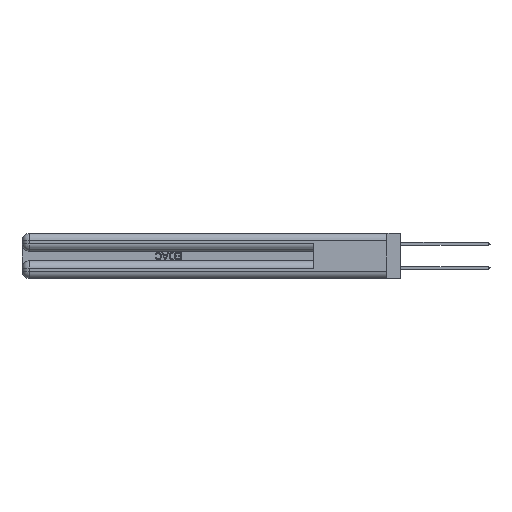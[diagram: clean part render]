
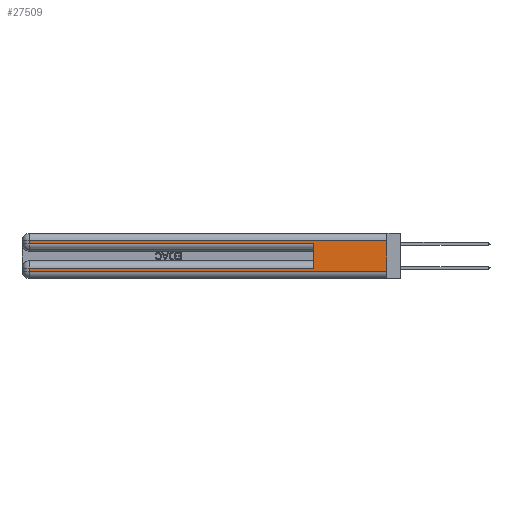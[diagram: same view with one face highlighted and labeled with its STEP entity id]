
A CAD part, left-side view. The second image highlights one B-rep face of the part: STEP entity #27509.
In plain terms, the highlighted planar face has unit normal (-1, 0, 0).
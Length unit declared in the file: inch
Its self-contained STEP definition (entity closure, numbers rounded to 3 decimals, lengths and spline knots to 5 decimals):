
#192 = VERTEX_POINT ( 'NONE', #6987 ) ;
#917 = ORIENTED_EDGE ( 'NONE', *, *, #10895, .T. ) ;
#2391 = CARTESIAN_POINT ( 'NONE',  ( 0., 0., 0.37 ) ) ;
#2930 = VERTEX_POINT ( 'NONE', #15470 ) ;
#3002 = CARTESIAN_POINT ( 'NONE',  ( 0., 0., 0.06 ) ) ;
#3645 = CARTESIAN_POINT ( 'NONE',  ( 0., 0., 0.31 ) ) ;
#3798 = ORIENTED_EDGE ( 'NONE', *, *, #39941, .F. ) ;
#5053 = VECTOR ( 'NONE', #23461, 39.37008 ) ;
#6502 = EDGE_CURVE ( 'NONE', #22265, #192, #21570, .T. ) ;
#6736 = VECTOR ( 'NONE', #7463, 39.37008 ) ;
#6833 = CARTESIAN_POINT ( 'NONE',  ( 0., 2.94, 0.37 ) ) ;
#6987 = CARTESIAN_POINT ( 'NONE',  ( 0., 2.94, 0.285 ) ) ;
#7341 = VERTEX_POINT ( 'NONE', #17289 ) ;
#7463 = DIRECTION ( 'NONE',  ( 0., 1., 0. ) ) ;
#7675 = CARTESIAN_POINT ( 'NONE',  ( 0., 2.94, 0.37 ) ) ;
#8107 = PLANE ( 'NONE',  #39879 ) ;
#8289 = EDGE_CURVE ( 'NONE', #192, #41478, #34525, .T. ) ;
#10895 = EDGE_CURVE ( 'NONE', #2930, #25895, #14862, .T. ) ;
#11434 = DIRECTION ( 'NONE',  ( 0., 0., -1. ) ) ;
#11670 = VECTOR ( 'NONE', #47206, 39.37008 ) ;
#13680 = VECTOR ( 'NONE', #32688, 39.37008 ) ;
#13960 = VERTEX_POINT ( 'NONE', #19303 ) ;
#14805 = ORIENTED_EDGE ( 'NONE', *, *, #6502, .T. ) ;
#14862 = LINE ( 'NONE', #3002, #13680 ) ;
#15470 = CARTESIAN_POINT ( 'NONE',  ( 0., 2.94, 0.06 ) ) ;
#15638 = CARTESIAN_POINT ( 'NONE',  ( 0., 0., 0.37 ) ) ;
#15807 = VECTOR ( 'NONE', #43833, 39.37008 ) ;
#17210 = EDGE_CURVE ( 'NONE', #13960, #41478, #32403, .T. ) ;
#17289 = CARTESIAN_POINT ( 'NONE',  ( 0., 0., 0.31 ) ) ;
#17436 = DIRECTION ( 'NONE',  ( 0., 0., 1. ) ) ;
#19303 = CARTESIAN_POINT ( 'NONE',  ( 0., 0.6, 0.085 ) ) ;
#19344 = DIRECTION ( 'NONE',  ( 1., 0., 0. ) ) ;
#19757 = CARTESIAN_POINT ( 'NONE',  ( 0., 0., 0.285 ) ) ;
#21570 = LINE ( 'NONE', #6833, #11670 ) ;
#22265 = VERTEX_POINT ( 'NONE', #40867 ) ;
#22826 = EDGE_CURVE ( 'NONE', #13960, #40471, #25610, .T. ) ;
#23461 = DIRECTION ( 'NONE',  ( 0., -1., 0. ) ) ;
#24745 = DIRECTION ( 'NONE',  ( 0., 0., -1. ) ) ;
#24899 = ORIENTED_EDGE ( 'NONE', *, *, #30903, .T. ) ;
#24969 = CARTESIAN_POINT ( 'NONE',  ( 0., 0.6, 0.145 ) ) ;
#25610 = LINE ( 'NONE', #32856, #15807 ) ;
#25895 = VERTEX_POINT ( 'NONE', #39810 ) ;
#27509 = ADVANCED_FACE ( 'NONE', ( #47168 ), #8107, .F. ) ;
#28100 = VECTOR ( 'NONE', #24745, 39.37008 ) ;
#29808 = LINE ( 'NONE', #7675, #38330 ) ;
#30903 = EDGE_CURVE ( 'NONE', #40471, #2930, #29808, .T. ) ;
#31263 = VECTOR ( 'NONE', #17436, 39.37008 ) ;
#32403 = LINE ( 'NONE', #24969, #31263 ) ;
#32688 = DIRECTION ( 'NONE',  ( 0., -1., 0. ) ) ;
#32705 = EDGE_LOOP ( 'NONE', ( #3798, #37897, #14805, #44655, #41698, #47774, #24899, #917 ) ) ;
#32856 = CARTESIAN_POINT ( 'NONE',  ( 0., 0., 0.085 ) ) ;
#34525 = LINE ( 'NONE', #19757, #5053 ) ;
#36173 = LINE ( 'NONE', #3645, #6736 ) ;
#36629 = LINE ( 'NONE', #2391, #28100 ) ;
#37897 = ORIENTED_EDGE ( 'NONE', *, *, #38825, .T. ) ;
#38330 = VECTOR ( 'NONE', #11434, 39.37008 ) ;
#38825 = EDGE_CURVE ( 'NONE', #7341, #22265, #36173, .T. ) ;
#39810 = CARTESIAN_POINT ( 'NONE',  ( 0., 0., 0.06 ) ) ;
#39879 = AXIS2_PLACEMENT_3D ( 'NONE', #15638, #19344, #44909 ) ;
#39941 = EDGE_CURVE ( 'NONE', #7341, #25895, #36629, .T. ) ;
#40471 = VERTEX_POINT ( 'NONE', #45754 ) ;
#40763 = CARTESIAN_POINT ( 'NONE',  ( 0., 0.6, 0.285 ) ) ;
#40867 = CARTESIAN_POINT ( 'NONE',  ( 0., 2.94, 0.31 ) ) ;
#41478 = VERTEX_POINT ( 'NONE', #40763 ) ;
#41698 = ORIENTED_EDGE ( 'NONE', *, *, #17210, .F. ) ;
#43833 = DIRECTION ( 'NONE',  ( 0., 1., 0. ) ) ;
#44655 = ORIENTED_EDGE ( 'NONE', *, *, #8289, .T. ) ;
#44909 = DIRECTION ( 'NONE',  ( 0., 0., -1. ) ) ;
#45754 = CARTESIAN_POINT ( 'NONE',  ( 0., 2.94, 0.085 ) ) ;
#47168 = FACE_OUTER_BOUND ( 'NONE', #32705, .T. ) ;
#47206 = DIRECTION ( 'NONE',  ( 0., 0., -1. ) ) ;
#47774 = ORIENTED_EDGE ( 'NONE', *, *, #22826, .T. ) ;
